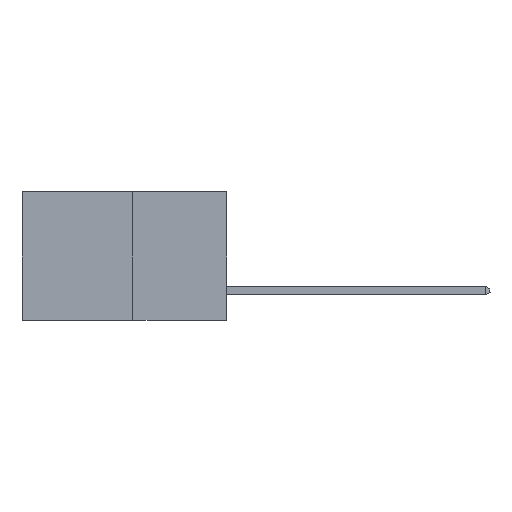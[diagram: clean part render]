
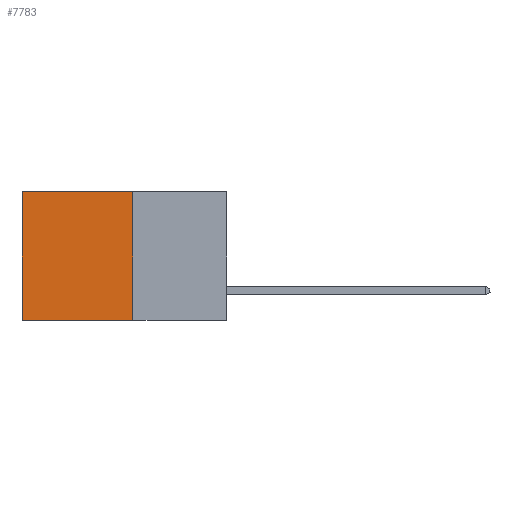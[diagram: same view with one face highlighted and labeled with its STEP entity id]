
A CAD part, left-side view. The second image highlights one B-rep face of the part: STEP entity #7783.
In plain terms, the highlighted planar face has unit normal (-1, 0, 0).
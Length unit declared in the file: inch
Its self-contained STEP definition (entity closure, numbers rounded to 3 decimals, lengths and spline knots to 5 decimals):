
#126 = DIRECTION ( 'NONE',  ( 0., 0., -1. ) ) ;
#765 = CARTESIAN_POINT ( 'NONE',  ( 0.277, 0.27, -0.37 ) ) ;
#1324 = CARTESIAN_POINT ( 'NONE',  ( 0.277, 0.59, -0.37 ) ) ;
#1659 = LINE ( 'NONE', #6598, #14409 ) ;
#2148 = CARTESIAN_POINT ( 'NONE',  ( 0.277, 0.27, -0.37 ) ) ;
#2621 = LINE ( 'NONE', #11705, #12100 ) ;
#3909 = EDGE_CURVE ( 'NONE', #13559, #11292, #11593, .T. ) ;
#3985 = ORIENTED_EDGE ( 'NONE', *, *, #15901, .F. ) ;
#4522 = EDGE_CURVE ( 'NONE', #6670, #15721, #1659, .T. ) ;
#4689 = ORIENTED_EDGE ( 'NONE', *, *, #5078, .T. ) ;
#5078 = EDGE_CURVE ( 'NONE', #15721, #11292, #2621, .T. ) ;
#5349 = ORIENTED_EDGE ( 'NONE', *, *, #3909, .F. ) ;
#5715 = EDGE_LOOP ( 'NONE', ( #4689, #5349, #3985, #5791 ) ) ;
#5791 = ORIENTED_EDGE ( 'NONE', *, *, #4522, .T. ) ;
#6389 = VECTOR ( 'NONE', #126, 39.37008 ) ;
#6598 = CARTESIAN_POINT ( 'NONE',  ( 0.277, 0.27, 0. ) ) ;
#6642 = DIRECTION ( 'NONE',  ( 0., 1., 0. ) ) ;
#6670 = VERTEX_POINT ( 'NONE', #14140 ) ;
#7783 = ADVANCED_FACE ( 'NONE', ( #13181 ), #12517, .F. ) ;
#8225 = VECTOR ( 'NONE', #12045, 39.37008 ) ;
#9829 = LINE ( 'NONE', #10544, #6389 ) ;
#9949 = AXIS2_PLACEMENT_3D ( 'NONE', #12642, #12516, #12499 ) ;
#10544 = CARTESIAN_POINT ( 'NONE',  ( 0.277, 0.27, -0.37 ) ) ;
#11292 = VERTEX_POINT ( 'NONE', #1324 ) ;
#11391 = DIRECTION ( 'NONE',  ( 0., 0., -1. ) ) ;
#11593 = LINE ( 'NONE', #2148, #8225 ) ;
#11705 = CARTESIAN_POINT ( 'NONE',  ( 0.277, 0.59, -0.37 ) ) ;
#12045 = DIRECTION ( 'NONE',  ( 0., 1., 0. ) ) ;
#12100 = VECTOR ( 'NONE', #11391, 39.37008 ) ;
#12499 = DIRECTION ( 'NONE',  ( 0., 0., -1. ) ) ;
#12516 = DIRECTION ( 'NONE',  ( 1., 0., 0. ) ) ;
#12517 = PLANE ( 'NONE',  #9949 ) ;
#12642 = CARTESIAN_POINT ( 'NONE',  ( 0.277, 0.27, -0.37 ) ) ;
#13181 = FACE_OUTER_BOUND ( 'NONE', #5715, .T. ) ;
#13559 = VERTEX_POINT ( 'NONE', #765 ) ;
#13886 = CARTESIAN_POINT ( 'NONE',  ( 0.277, 0.59, 0. ) ) ;
#14140 = CARTESIAN_POINT ( 'NONE',  ( 0.277, 0.27, 0. ) ) ;
#14409 = VECTOR ( 'NONE', #6642, 39.37008 ) ;
#15721 = VERTEX_POINT ( 'NONE', #13886 ) ;
#15901 = EDGE_CURVE ( 'NONE', #6670, #13559, #9829, .T. ) ;
